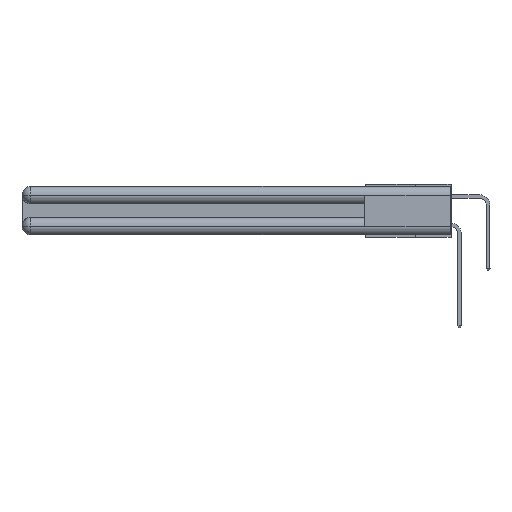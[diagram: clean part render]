
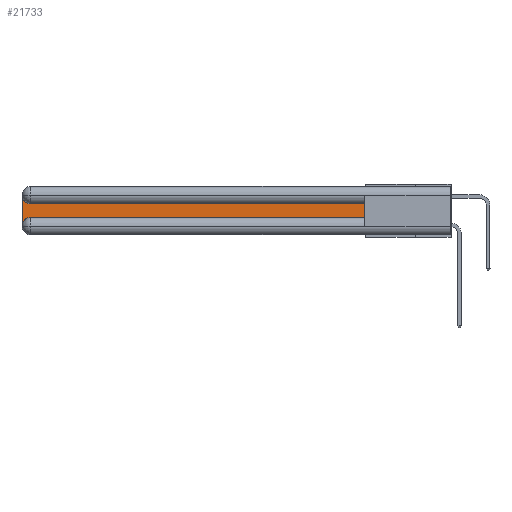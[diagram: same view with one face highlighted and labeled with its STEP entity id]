
A CAD part, left-side view. The second image highlights one B-rep face of the part: STEP entity #21733.
In plain terms, the highlighted planar face has unit normal (-1, 0, 0).
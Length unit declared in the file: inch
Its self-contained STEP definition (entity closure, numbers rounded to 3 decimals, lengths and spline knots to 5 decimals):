
#723 = EDGE_CURVE ( 'NONE', #31629, #11769, #12006, .T. ) ;
#1289 = LINE ( 'NONE', #9804, #31290 ) ;
#2696 = CARTESIAN_POINT ( 'NONE',  ( 0.075, 0.6, -0.2175 ) ) ;
#2823 = AXIS2_PLACEMENT_3D ( 'NONE', #30075, #7133, #12507 ) ;
#4295 = EDGE_CURVE ( 'NONE', #26077, #14150, #8210, .T. ) ;
#4898 = DIRECTION ( 'NONE',  ( 0., 0., 1. ) ) ;
#5113 = ORIENTED_EDGE ( 'NONE', *, *, #8656, .T. ) ;
#5524 = ORIENTED_EDGE ( 'NONE', *, *, #4295, .T. ) ;
#5769 = VECTOR ( 'NONE', #19390, 39.37008 ) ;
#6573 = CARTESIAN_POINT ( 'NONE',  ( 0.075, 0.6, -0.2175 ) ) ;
#7133 = DIRECTION ( 'NONE',  ( 1., 0., 0. ) ) ;
#8210 = CIRCLE ( 'NONE', #32012, 0.06 ) ;
#8512 = CARTESIAN_POINT ( 'NONE',  ( 0.075, 0.6, -0.1225 ) ) ;
#8656 = EDGE_CURVE ( 'NONE', #14150, #31629, #1289, .T. ) ;
#9804 = CARTESIAN_POINT ( 'NONE',  ( 0.075, 3., -0.2175 ) ) ;
#9940 = ORIENTED_EDGE ( 'NONE', *, *, #723, .T. ) ;
#10173 = CARTESIAN_POINT ( 'NONE',  ( 0.075, 2.94, -0.0625 ) ) ;
#10703 = ORIENTED_EDGE ( 'NONE', *, *, #23979, .T. ) ;
#11085 = VERTEX_POINT ( 'NONE', #22610 ) ;
#11315 = CARTESIAN_POINT ( 'NONE',  ( 0.075, 3., -0.2775 ) ) ;
#11769 = VERTEX_POINT ( 'NONE', #15287 ) ;
#12006 = CIRCLE ( 'NONE', #2823, 0.06 ) ;
#12507 = DIRECTION ( 'NONE',  ( 0., 0., -1. ) ) ;
#12626 = CARTESIAN_POINT ( 'NONE',  ( 0.075, 2.94, -0.1225 ) ) ;
#12715 = VERTEX_POINT ( 'NONE', #8512 ) ;
#12780 = ORIENTED_EDGE ( 'NONE', *, *, #32149, .T. ) ;
#12883 = EDGE_CURVE ( 'NONE', #11769, #11085, #17451, .T. ) ;
#13053 = LINE ( 'NONE', #32510, #17488 ) ;
#13375 = PLANE ( 'NONE',  #29725 ) ;
#13779 = FACE_OUTER_BOUND ( 'NONE', #28119, .T. ) ;
#14150 = VERTEX_POINT ( 'NONE', #17007 ) ;
#14857 = DIRECTION ( 'NONE',  ( 0., 0., -1. ) ) ;
#15287 = CARTESIAN_POINT ( 'NONE',  ( 0.075, 2.94, -0.2175 ) ) ;
#15873 = CARTESIAN_POINT ( 'NONE',  ( 0.075, 3., -0.1225 ) ) ;
#16798 = DIRECTION ( 'NONE',  ( 0., 1., 0. ) ) ;
#17007 = CARTESIAN_POINT ( 'NONE',  ( 0.075, 3., -0.0625 ) ) ;
#17451 = LINE ( 'NONE', #6573, #5769 ) ;
#17488 = VECTOR ( 'NONE', #16798, 39.37008 ) ;
#17601 = DIRECTION ( 'NONE',  ( 0., 0., -1. ) ) ;
#18157 = VECTOR ( 'NONE', #4898, 39.37008 ) ;
#19390 = DIRECTION ( 'NONE',  ( 0., -1., 0. ) ) ;
#20409 = ORIENTED_EDGE ( 'NONE', *, *, #12883, .T. ) ;
#21733 = ADVANCED_FACE ( 'NONE', ( #13779 ), #13375, .F. ) ;
#22610 = CARTESIAN_POINT ( 'NONE',  ( 0.075, 0.6, -0.2175 ) ) ;
#23979 = EDGE_CURVE ( 'NONE', #12715, #26077, #13053, .T. ) ;
#24884 = LINE ( 'NONE', #2696, #18157 ) ;
#25668 = DIRECTION ( 'NONE',  ( 1., 0., 0. ) ) ;
#26077 = VERTEX_POINT ( 'NONE', #12626 ) ;
#28119 = EDGE_LOOP ( 'NONE', ( #10703, #5524, #5113, #9940, #20409, #12780 ) ) ;
#29725 = AXIS2_PLACEMENT_3D ( 'NONE', #15873, #25668, #31300 ) ;
#30075 = CARTESIAN_POINT ( 'NONE',  ( 0.075, 2.94, -0.2775 ) ) ;
#31290 = VECTOR ( 'NONE', #14857, 39.37008 ) ;
#31300 = DIRECTION ( 'NONE',  ( 0., 0., -1. ) ) ;
#31629 = VERTEX_POINT ( 'NONE', #11315 ) ;
#32012 = AXIS2_PLACEMENT_3D ( 'NONE', #10173, #32881, #17601 ) ;
#32149 = EDGE_CURVE ( 'NONE', #11085, #12715, #24884, .T. ) ;
#32510 = CARTESIAN_POINT ( 'NONE',  ( 0.075, 0.6, -0.1225 ) ) ;
#32881 = DIRECTION ( 'NONE',  ( 1., 0., 0. ) ) ;
